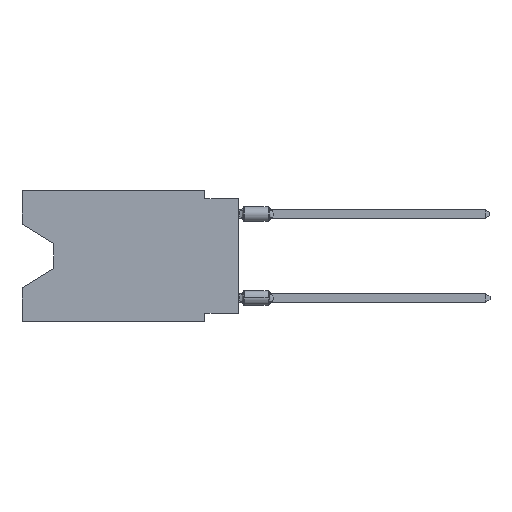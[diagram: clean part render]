
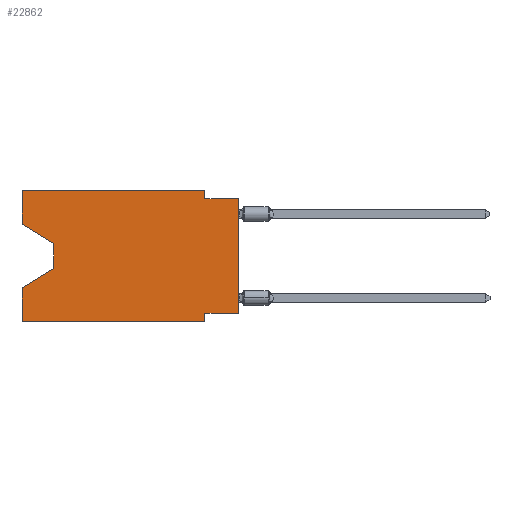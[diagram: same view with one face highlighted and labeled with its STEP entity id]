
A CAD part, left-side view. The second image highlights one B-rep face of the part: STEP entity #22862.
In plain terms, the highlighted planar face has unit normal (-1, 0, 0).
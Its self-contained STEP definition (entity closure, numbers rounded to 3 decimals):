
#1243 = VECTOR ( 'NONE', #11626, 1000. ) ;
#1304 = EDGE_CURVE ( 'NONE', #15910, #26495, #14979, .T. ) ;
#1531 = CARTESIAN_POINT ( 'NONE',  ( 0., 13.97, -4.013 ) ) ;
#1688 = VECTOR ( 'NONE', #7261, 1000. ) ;
#1940 = CARTESIAN_POINT ( 'NONE',  ( 0., 2.54, -0.635 ) ) ;
#2083 = VECTOR ( 'NONE', #16431, 1000. ) ;
#2125 = CARTESIAN_POINT ( 'NONE',  ( 0., 2.54, 0. ) ) ;
#2243 = VERTEX_POINT ( 'NONE', #22983 ) ;
#2297 = ORIENTED_EDGE ( 'NONE', *, *, #21948, .F. ) ;
#2384 = CARTESIAN_POINT ( 'NONE',  ( 0., 16.383, -9.906 ) ) ;
#2607 = VERTEX_POINT ( 'NONE', #18587 ) ;
#3014 = CARTESIAN_POINT ( 'NONE',  ( 0., 16.383, -9.906 ) ) ;
#3297 = CARTESIAN_POINT ( 'NONE',  ( 0., 0., -0.635 ) ) ;
#3549 = DIRECTION ( 'NONE',  ( 0., 0., -1. ) ) ;
#3981 = DIRECTION ( 'NONE',  ( 0., 0., 1. ) ) ;
#4051 = DIRECTION ( 'NONE',  ( 0., 0., -1. ) ) ;
#4422 = CARTESIAN_POINT ( 'NONE',  ( 0., 0., 0. ) ) ;
#4743 = VERTEX_POINT ( 'NONE', #1531 ) ;
#5078 = VECTOR ( 'NONE', #11592, 1000. ) ;
#5482 = VECTOR ( 'NONE', #13815, 1000. ) ;
#5770 = CARTESIAN_POINT ( 'NONE',  ( 0., 2.54, -9.271 ) ) ;
#6568 = CARTESIAN_POINT ( 'NONE',  ( 0., 0., -9.271 ) ) ;
#6602 = ORIENTED_EDGE ( 'NONE', *, *, #9513, .F. ) ;
#6773 = ORIENTED_EDGE ( 'NONE', *, *, #1304, .F. ) ;
#6789 = VERTEX_POINT ( 'NONE', #5770 ) ;
#7261 = DIRECTION ( 'NONE',  ( 0., -0.855, -0.519 ) ) ;
#7465 = CARTESIAN_POINT ( 'NONE',  ( 0., 16.383, -2.546 ) ) ;
#7754 = VECTOR ( 'NONE', #3981, 1000. ) ;
#7949 = CARTESIAN_POINT ( 'NONE',  ( 0., 13.97, -5.893 ) ) ;
#8340 = EDGE_CURVE ( 'NONE', #9334, #4743, #17919, .T. ) ;
#8358 = FACE_OUTER_BOUND ( 'NONE', #18909, .T. ) ;
#8398 = EDGE_CURVE ( 'NONE', #19279, #2607, #22010, .T. ) ;
#8584 = ORIENTED_EDGE ( 'NONE', *, *, #10806, .T. ) ;
#9334 = VERTEX_POINT ( 'NONE', #7465 ) ;
#9404 = CARTESIAN_POINT ( 'NONE',  ( 0., 0., -9.271 ) ) ;
#9513 = EDGE_CURVE ( 'NONE', #9334, #15910, #22701, .T. ) ;
#10014 = LINE ( 'NONE', #7949, #5482 ) ;
#10637 = ORIENTED_EDGE ( 'NONE', *, *, #8340, .T. ) ;
#10806 = EDGE_CURVE ( 'NONE', #11660, #14957, #13246, .T. ) ;
#10969 = EDGE_CURVE ( 'NONE', #26495, #19279, #17745, .T. ) ;
#11087 = VECTOR ( 'NONE', #25967, 1000. ) ;
#11592 = DIRECTION ( 'NONE',  ( 0., 1., 0. ) ) ;
#11621 = CARTESIAN_POINT ( 'NONE',  ( 0., 16.383, 0. ) ) ;
#11626 = DIRECTION ( 'NONE',  ( 0., -1., 0. ) ) ;
#11660 = VERTEX_POINT ( 'NONE', #2384 ) ;
#12320 = CARTESIAN_POINT ( 'NONE',  ( 0., 16.383, 0. ) ) ;
#12533 = DIRECTION ( 'NONE',  ( 0., -1., 0. ) ) ;
#12614 = ORIENTED_EDGE ( 'NONE', *, *, #19239, .T. ) ;
#12794 = ORIENTED_EDGE ( 'NONE', *, *, #10969, .F. ) ;
#13201 = ORIENTED_EDGE ( 'NONE', *, *, #23731, .T. ) ;
#13246 = LINE ( 'NONE', #3014, #26145 ) ;
#13815 = DIRECTION ( 'NONE',  ( 0., 0.855, -0.519 ) ) ;
#13956 = CARTESIAN_POINT ( 'NONE',  ( 0., 16.383, 0. ) ) ;
#14497 = DIRECTION ( 'NONE',  ( 1., 0., 0. ) ) ;
#14695 = ORIENTED_EDGE ( 'NONE', *, *, #8398, .F. ) ;
#14786 = CARTESIAN_POINT ( 'NONE',  ( 0., 13.97, -5.893 ) ) ;
#14861 = VERTEX_POINT ( 'NONE', #6568 ) ;
#14957 = VERTEX_POINT ( 'NONE', #21593 ) ;
#14979 = LINE ( 'NONE', #18699, #25639 ) ;
#15235 = AXIS2_PLACEMENT_3D ( 'NONE', #12320, #14497, #22430 ) ;
#15416 = DIRECTION ( 'NONE',  ( 0., -1., 0. ) ) ;
#15910 = VERTEX_POINT ( 'NONE', #13956 ) ;
#15962 = LINE ( 'NONE', #11621, #11087 ) ;
#16431 = DIRECTION ( 'NONE',  ( 0., 0., 1. ) ) ;
#16839 = VECTOR ( 'NONE', #22728, 1000. ) ;
#17745 = LINE ( 'NONE', #22262, #23114 ) ;
#17919 = LINE ( 'NONE', #19840, #1688 ) ;
#18137 = EDGE_CURVE ( 'NONE', #21376, #2243, #10014, .T. ) ;
#18201 = CARTESIAN_POINT ( 'NONE',  ( 0., 13.97, -4.013 ) ) ;
#18587 = CARTESIAN_POINT ( 'NONE',  ( 0., 0., -0.635 ) ) ;
#18699 = CARTESIAN_POINT ( 'NONE',  ( 0., 16.383, 0. ) ) ;
#18888 = EDGE_CURVE ( 'NONE', #14861, #6789, #21975, .T. ) ;
#18909 = EDGE_LOOP ( 'NONE', ( #10637, #12614, #22677, #19952, #8584, #2297, #25494, #13201, #14695, #12794, #6773, #6602 ) ) ;
#19239 = EDGE_CURVE ( 'NONE', #4743, #21376, #20394, .T. ) ;
#19279 = VERTEX_POINT ( 'NONE', #1940 ) ;
#19840 = CARTESIAN_POINT ( 'NONE',  ( 0., 16.383, -2.546 ) ) ;
#19952 = ORIENTED_EDGE ( 'NONE', *, *, #24348, .F. ) ;
#20394 = LINE ( 'NONE', #18201, #16839 ) ;
#20770 = CARTESIAN_POINT ( 'NONE',  ( 0., 16.383, 0. ) ) ;
#21376 = VERTEX_POINT ( 'NONE', #14786 ) ;
#21593 = CARTESIAN_POINT ( 'NONE',  ( 0., 2.54, -9.906 ) ) ;
#21948 = EDGE_CURVE ( 'NONE', #6789, #14957, #23168, .T. ) ;
#21975 = LINE ( 'NONE', #9404, #5078 ) ;
#22010 = LINE ( 'NONE', #3297, #1243 ) ;
#22262 = CARTESIAN_POINT ( 'NONE',  ( 0., 2.54, 0. ) ) ;
#22430 = DIRECTION ( 'NONE',  ( 0., 0., -1. ) ) ;
#22566 = PLANE ( 'NONE',  #15235 ) ;
#22677 = ORIENTED_EDGE ( 'NONE', *, *, #18137, .T. ) ;
#22701 = LINE ( 'NONE', #20770, #7754 ) ;
#22728 = DIRECTION ( 'NONE',  ( 0., 0., -1. ) ) ;
#22862 = ADVANCED_FACE ( 'NONE', ( #8358 ), #22566, .F. ) ;
#22897 = CARTESIAN_POINT ( 'NONE',  ( 0., 2.54, -9.906 ) ) ;
#22983 = CARTESIAN_POINT ( 'NONE',  ( 0., 16.383, -7.36 ) ) ;
#23114 = VECTOR ( 'NONE', #3549, 1000. ) ;
#23140 = LINE ( 'NONE', #4422, #2083 ) ;
#23168 = LINE ( 'NONE', #22897, #25237 ) ;
#23731 = EDGE_CURVE ( 'NONE', #14861, #2607, #23140, .T. ) ;
#24348 = EDGE_CURVE ( 'NONE', #11660, #2243, #15962, .T. ) ;
#25237 = VECTOR ( 'NONE', #4051, 1000. ) ;
#25494 = ORIENTED_EDGE ( 'NONE', *, *, #18888, .F. ) ;
#25639 = VECTOR ( 'NONE', #12533, 1000. ) ;
#25967 = DIRECTION ( 'NONE',  ( 0., 0., 1. ) ) ;
#26145 = VECTOR ( 'NONE', #15416, 1000. ) ;
#26495 = VERTEX_POINT ( 'NONE', #2125 ) ;
